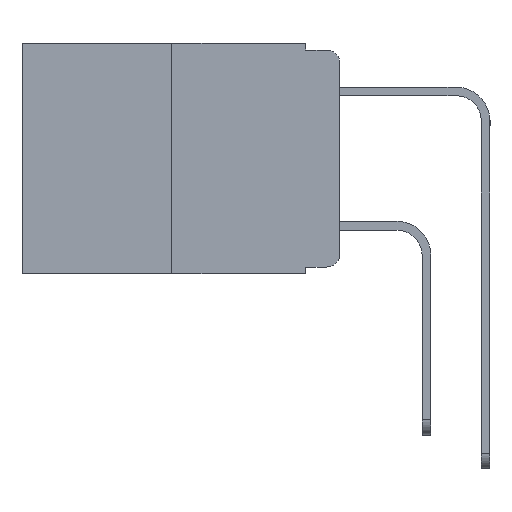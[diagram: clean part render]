
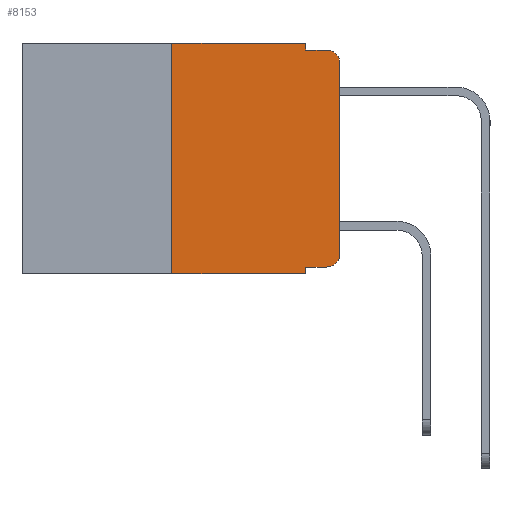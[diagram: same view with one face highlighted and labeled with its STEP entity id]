
A CAD part, left-side view. The second image highlights one B-rep face of the part: STEP entity #8153.
In plain terms, the highlighted planar face has unit normal (-1, 0, 0).
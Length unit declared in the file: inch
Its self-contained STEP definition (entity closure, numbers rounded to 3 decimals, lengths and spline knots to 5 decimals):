
#162 = DIRECTION ( 'NONE',  ( 0., -1., 0. ) ) ;
#388 = CARTESIAN_POINT ( 'NONE',  ( 0., 0.02, -0.333 ) ) ;
#485 = VERTEX_POINT ( 'NONE', #9557 ) ;
#563 = DIRECTION ( 'NONE',  ( -1., 0., 0. ) ) ;
#602 = EDGE_CURVE ( 'NONE', #11421, #10036, #10867, .T. ) ;
#1094 = CARTESIAN_POINT ( 'NONE',  ( 0., 0., -0.313 ) ) ;
#1108 = VECTOR ( 'NONE', #9137, 39.37008 ) ;
#1114 = DIRECTION ( 'NONE',  ( 0., 0., -1. ) ) ;
#1135 = CARTESIAN_POINT ( 'NONE',  ( 0., 0.25, 0. ) ) ;
#1212 = EDGE_CURVE ( 'NONE', #11389, #10115, #9229, .T. ) ;
#1339 = DIRECTION ( 'NONE',  ( 0., -1., 0. ) ) ;
#2367 = CARTESIAN_POINT ( 'NONE',  ( 0., 0.051, -0.333 ) ) ;
#2461 = CIRCLE ( 'NONE', #10579, 0.02 ) ;
#2619 = LINE ( 'NONE', #12052, #8004 ) ;
#2690 = EDGE_CURVE ( 'NONE', #10036, #10150, #2461, .T. ) ;
#3023 = EDGE_CURVE ( 'NONE', #5828, #11421, #12332, .T. ) ;
#3087 = VERTEX_POINT ( 'NONE', #3413 ) ;
#3162 = ORIENTED_EDGE ( 'NONE', *, *, #1212, .F. ) ;
#3305 = VERTEX_POINT ( 'NONE', #10112 ) ;
#3386 = LINE ( 'NONE', #2367, #11210 ) ;
#3413 = CARTESIAN_POINT ( 'NONE',  ( 0., 0.051, -0.333 ) ) ;
#3735 = ORIENTED_EDGE ( 'NONE', *, *, #7273, .F. ) ;
#4108 = ORIENTED_EDGE ( 'NONE', *, *, #2690, .T. ) ;
#4113 = EDGE_LOOP ( 'NONE', ( #8572, #4108, #3735, #11995, #5265, #3162, #11734, #5643, #6320, #11902 ) ) ;
#4225 = DIRECTION ( 'NONE',  ( 0., -1., 0. ) ) ;
#4302 = FACE_OUTER_BOUND ( 'NONE', #4113, .T. ) ;
#5192 = EDGE_CURVE ( 'NONE', #3087, #5828, #3386, .T. ) ;
#5223 = VECTOR ( 'NONE', #8687, 39.37008 ) ;
#5265 = ORIENTED_EDGE ( 'NONE', *, *, #13234, .F. ) ;
#5418 = PLANE ( 'NONE',  #11434 ) ;
#5450 = CARTESIAN_POINT ( 'NONE',  ( 0., 0.02, -0.313 ) ) ;
#5476 = VECTOR ( 'NONE', #13586, 39.37008 ) ;
#5562 = CARTESIAN_POINT ( 'NONE',  ( 0., 0., 0. ) ) ;
#5643 = ORIENTED_EDGE ( 'NONE', *, *, #8787, .F. ) ;
#5828 = VERTEX_POINT ( 'NONE', #388 ) ;
#6131 = LINE ( 'NONE', #11640, #11423 ) ;
#6298 = CARTESIAN_POINT ( 'NONE',  ( 0., 0.02, -0.01 ) ) ;
#6320 = ORIENTED_EDGE ( 'NONE', *, *, #5192, .T. ) ;
#6451 = CARTESIAN_POINT ( 'NONE',  ( 0., 0.051, 0. ) ) ;
#6494 = DIRECTION ( 'NONE',  ( 0., 0., -1. ) ) ;
#7038 = CARTESIAN_POINT ( 'NONE',  ( 0., 0.02, -0.03 ) ) ;
#7273 = EDGE_CURVE ( 'NONE', #11577, #10150, #12367, .T. ) ;
#7287 = CARTESIAN_POINT ( 'NONE',  ( 0., 0.25, 0. ) ) ;
#7559 = DIRECTION ( 'NONE',  ( 1., 0., 0. ) ) ;
#8004 = VECTOR ( 'NONE', #13001, 39.37008 ) ;
#8072 = CARTESIAN_POINT ( 'NONE',  ( 0., 0.051, -0.01 ) ) ;
#8130 = DIRECTION ( 'NONE',  ( 0., 0., -1. ) ) ;
#8153 = ADVANCED_FACE ( 'NONE', ( #4302 ), #5418, .F. ) ;
#8209 = LINE ( 'NONE', #10915, #13264 ) ;
#8239 = AXIS2_PLACEMENT_3D ( 'NONE', #5450, #12708, #6494 ) ;
#8249 = CARTESIAN_POINT ( 'NONE',  ( 0., 0., -0.03 ) ) ;
#8572 = ORIENTED_EDGE ( 'NONE', *, *, #602, .T. ) ;
#8687 = DIRECTION ( 'NONE',  ( 0., 0., 1. ) ) ;
#8722 = EDGE_CURVE ( 'NONE', #11389, #485, #6131, .T. ) ;
#8787 = EDGE_CURVE ( 'NONE', #3087, #485, #13070, .T. ) ;
#8902 = CARTESIAN_POINT ( 'NONE',  ( 0., 0.051, -0.01 ) ) ;
#8989 = EDGE_CURVE ( 'NONE', #3305, #11577, #2619, .T. ) ;
#9137 = DIRECTION ( 'NONE',  ( 0., -1., 0. ) ) ;
#9229 = LINE ( 'NONE', #1135, #11956 ) ;
#9557 = CARTESIAN_POINT ( 'NONE',  ( 0., 0.051, -0.343 ) ) ;
#9675 = DIRECTION ( 'NONE',  ( 0., 0., 1. ) ) ;
#10036 = VERTEX_POINT ( 'NONE', #8249 ) ;
#10112 = CARTESIAN_POINT ( 'NONE',  ( 0., 0.051, 0. ) ) ;
#10115 = VERTEX_POINT ( 'NONE', #7287 ) ;
#10150 = VERTEX_POINT ( 'NONE', #6298 ) ;
#10579 = AXIS2_PLACEMENT_3D ( 'NONE', #7038, #563, #8130 ) ;
#10867 = LINE ( 'NONE', #5562, #5223 ) ;
#10915 = CARTESIAN_POINT ( 'NONE',  ( 0., 0.473, 0. ) ) ;
#11210 = VECTOR ( 'NONE', #1339, 39.37008 ) ;
#11389 = VERTEX_POINT ( 'NONE', #12625 ) ;
#11421 = VERTEX_POINT ( 'NONE', #1094 ) ;
#11423 = VECTOR ( 'NONE', #4225, 39.37008 ) ;
#11434 = AXIS2_PLACEMENT_3D ( 'NONE', #13642, #7559, #1114 ) ;
#11577 = VERTEX_POINT ( 'NONE', #8902 ) ;
#11640 = CARTESIAN_POINT ( 'NONE',  ( 0., 0.473, -0.343 ) ) ;
#11734 = ORIENTED_EDGE ( 'NONE', *, *, #8722, .T. ) ;
#11902 = ORIENTED_EDGE ( 'NONE', *, *, #3023, .T. ) ;
#11956 = VECTOR ( 'NONE', #9675, 39.37008 ) ;
#11995 = ORIENTED_EDGE ( 'NONE', *, *, #8989, .F. ) ;
#12052 = CARTESIAN_POINT ( 'NONE',  ( 0., 0.051, 0. ) ) ;
#12332 = CIRCLE ( 'NONE', #8239, 0.02 ) ;
#12367 = LINE ( 'NONE', #8072, #1108 ) ;
#12625 = CARTESIAN_POINT ( 'NONE',  ( 0., 0.25, -0.343 ) ) ;
#12708 = DIRECTION ( 'NONE',  ( -1., 0., 0. ) ) ;
#13001 = DIRECTION ( 'NONE',  ( 0., 0., -1. ) ) ;
#13070 = LINE ( 'NONE', #6451, #5476 ) ;
#13234 = EDGE_CURVE ( 'NONE', #10115, #3305, #8209, .T. ) ;
#13264 = VECTOR ( 'NONE', #162, 39.37008 ) ;
#13586 = DIRECTION ( 'NONE',  ( 0., 0., -1. ) ) ;
#13642 = CARTESIAN_POINT ( 'NONE',  ( 0., 0.473, 0. ) ) ;
